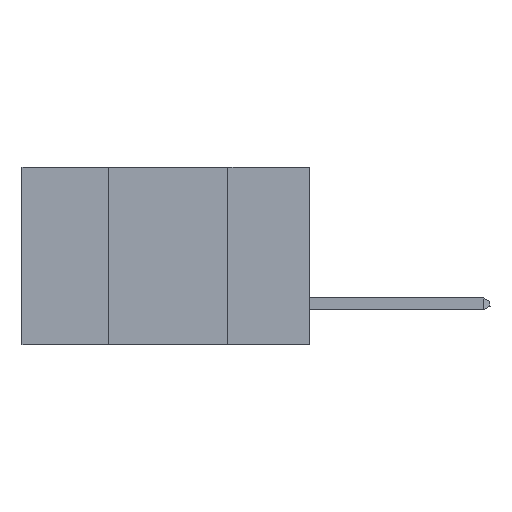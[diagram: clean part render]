
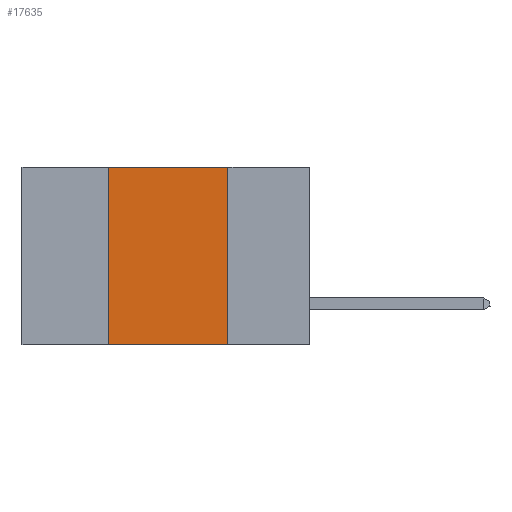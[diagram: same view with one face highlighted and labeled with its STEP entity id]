
A CAD part, left-side view. The second image highlights one B-rep face of the part: STEP entity #17635.
In plain terms, the highlighted planar face has unit normal (-1, 0, 0).
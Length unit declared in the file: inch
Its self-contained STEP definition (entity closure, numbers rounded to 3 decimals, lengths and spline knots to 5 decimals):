
#107 = ORIENTED_EDGE ( 'NONE', *, *, #31872, .T. ) ;
#211 = CARTESIAN_POINT ( 'NONE',  ( 0., 0.17, 0. ) ) ;
#1522 = DIRECTION ( 'NONE',  ( 0., -1., 0. ) ) ;
#2018 = AXIS2_PLACEMENT_3D ( 'NONE', #41081, #22382, #26081 ) ;
#7717 = PLANE ( 'NONE',  #2018 ) ;
#7726 = LINE ( 'NONE', #37419, #30118 ) ;
#9707 = VECTOR ( 'NONE', #29683, 39.37008 ) ;
#11795 = DIRECTION ( 'NONE',  ( 0., 0., 1. ) ) ;
#11981 = LINE ( 'NONE', #24789, #14293 ) ;
#12552 = CARTESIAN_POINT ( 'NONE',  ( 0., 0.42, 0. ) ) ;
#14293 = VECTOR ( 'NONE', #43192, 39.37008 ) ;
#15696 = VERTEX_POINT ( 'NONE', #12552 ) ;
#15860 = CARTESIAN_POINT ( 'NONE',  ( 0., 0.6, -0.37 ) ) ;
#16948 = EDGE_CURVE ( 'NONE', #26728, #21077, #45474, .T. ) ;
#17635 = ADVANCED_FACE ( 'NONE', ( #45381 ), #7717, .F. ) ;
#21077 = VERTEX_POINT ( 'NONE', #37042 ) ;
#22382 = DIRECTION ( 'NONE',  ( 1., 0., 0. ) ) ;
#24617 = CARTESIAN_POINT ( 'NONE',  ( 0., 0.17, 0. ) ) ;
#24731 = EDGE_CURVE ( 'NONE', #15696, #26728, #11981, .T. ) ;
#24789 = CARTESIAN_POINT ( 'NONE',  ( 0., 0.6, 0. ) ) ;
#26081 = DIRECTION ( 'NONE',  ( 0., 0., -1. ) ) ;
#26728 = VERTEX_POINT ( 'NONE', #24617 ) ;
#26952 = EDGE_LOOP ( 'NONE', ( #38460, #35862, #33987, #107 ) ) ;
#29683 = DIRECTION ( 'NONE',  ( 0., 0., -1. ) ) ;
#30118 = VECTOR ( 'NONE', #11795, 39.37008 ) ;
#30381 = VERTEX_POINT ( 'NONE', #39992 ) ;
#31872 = EDGE_CURVE ( 'NONE', #30381, #21077, #35175, .T. ) ;
#33987 = ORIENTED_EDGE ( 'NONE', *, *, #41060, .F. ) ;
#35175 = LINE ( 'NONE', #15860, #37485 ) ;
#35862 = ORIENTED_EDGE ( 'NONE', *, *, #24731, .F. ) ;
#37042 = CARTESIAN_POINT ( 'NONE',  ( 0., 0.17, -0.37 ) ) ;
#37419 = CARTESIAN_POINT ( 'NONE',  ( 0., 0.42, 0. ) ) ;
#37485 = VECTOR ( 'NONE', #1522, 39.37008 ) ;
#38460 = ORIENTED_EDGE ( 'NONE', *, *, #16948, .F. ) ;
#39992 = CARTESIAN_POINT ( 'NONE',  ( 0., 0.42, -0.37 ) ) ;
#41060 = EDGE_CURVE ( 'NONE', #30381, #15696, #7726, .T. ) ;
#41081 = CARTESIAN_POINT ( 'NONE',  ( 0., 0.6, 0. ) ) ;
#43192 = DIRECTION ( 'NONE',  ( 0., -1., 0. ) ) ;
#45381 = FACE_OUTER_BOUND ( 'NONE', #26952, .T. ) ;
#45474 = LINE ( 'NONE', #211, #9707 ) ;
